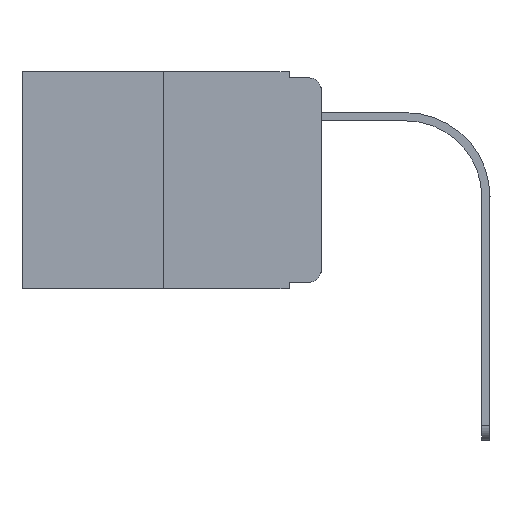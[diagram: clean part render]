
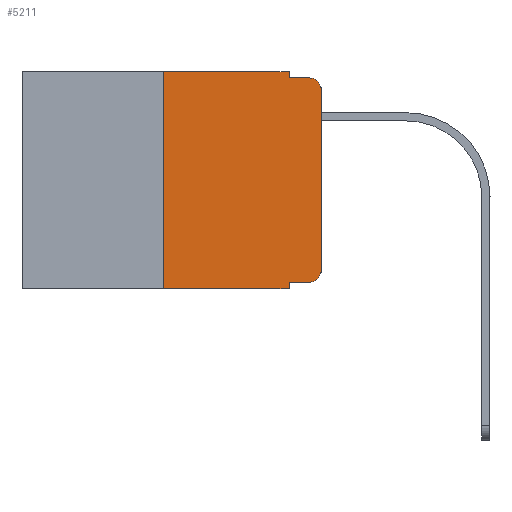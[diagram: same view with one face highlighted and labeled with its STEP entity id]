
A CAD part, left-side view. The second image highlights one B-rep face of the part: STEP entity #5211.
In plain terms, the highlighted planar face has unit normal (-1, 0, 0).
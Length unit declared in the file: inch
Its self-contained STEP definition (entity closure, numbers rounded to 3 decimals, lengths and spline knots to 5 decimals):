
#440 = CARTESIAN_POINT ( 'NONE',  ( 0., 0., -0.313 ) ) ;
#561 = AXIS2_PLACEMENT_3D ( 'NONE', #17655, #1024, #12655 ) ;
#601 = ORIENTED_EDGE ( 'NONE', *, *, #14092, .F. ) ;
#818 = VERTEX_POINT ( 'NONE', #8046 ) ;
#1024 = DIRECTION ( 'NONE',  ( -1., 0., 0. ) ) ;
#1051 = CARTESIAN_POINT ( 'NONE',  ( 0., 0., 0. ) ) ;
#1180 = CARTESIAN_POINT ( 'NONE',  ( 0., 0.473, -0.343 ) ) ;
#1638 = LINE ( 'NONE', #8075, #19813 ) ;
#1722 = DIRECTION ( 'NONE',  ( 0., -1., 0. ) ) ;
#1746 = PLANE ( 'NONE',  #20336 ) ;
#2055 = VECTOR ( 'NONE', #1722, 39.37008 ) ;
#2069 = CIRCLE ( 'NONE', #20827, 0.02 ) ;
#2169 = DIRECTION ( 'NONE',  ( -1., 0., 0. ) ) ;
#2252 = EDGE_CURVE ( 'NONE', #14280, #4525, #1638, .T. ) ;
#2274 = DIRECTION ( 'NONE',  ( 0., 0., -1. ) ) ;
#2506 = ORIENTED_EDGE ( 'NONE', *, *, #7189, .F. ) ;
#2559 = VERTEX_POINT ( 'NONE', #4293 ) ;
#2685 = CIRCLE ( 'NONE', #561, 0.02 ) ;
#2992 = CARTESIAN_POINT ( 'NONE',  ( 0., 0.02, -0.01 ) ) ;
#3070 = LINE ( 'NONE', #1180, #16499 ) ;
#3268 = ORIENTED_EDGE ( 'NONE', *, *, #11568, .T. ) ;
#3334 = VERTEX_POINT ( 'NONE', #2992 ) ;
#3627 = DIRECTION ( 'NONE',  ( 1., 0., 0. ) ) ;
#3714 = DIRECTION ( 'NONE',  ( 0., -1., 0. ) ) ;
#4293 = CARTESIAN_POINT ( 'NONE',  ( 0., 0.051, -0.333 ) ) ;
#4525 = VERTEX_POINT ( 'NONE', #16077 ) ;
#4785 = LINE ( 'NONE', #19764, #8509 ) ;
#5066 = FACE_OUTER_BOUND ( 'NONE', #5644, .T. ) ;
#5211 = ADVANCED_FACE ( 'NONE', ( #5066 ), #1746, .F. ) ;
#5538 = VECTOR ( 'NONE', #21335, 39.37008 ) ;
#5597 = VECTOR ( 'NONE', #10982, 39.37008 ) ;
#5644 = EDGE_LOOP ( 'NONE', ( #15351, #9209, #18653, #2506, #6189, #14084, #3268, #601, #20754, #16075 ) ) ;
#6189 = ORIENTED_EDGE ( 'NONE', *, *, #18873, .F. ) ;
#6763 = VERTEX_POINT ( 'NONE', #13357 ) ;
#7189 = EDGE_CURVE ( 'NONE', #19261, #6763, #21232, .T. ) ;
#7575 = VERTEX_POINT ( 'NONE', #15999 ) ;
#7802 = DIRECTION ( 'NONE',  ( 0., 0., 1. ) ) ;
#8043 = CARTESIAN_POINT ( 'NONE',  ( 0., 0.051, -0.333 ) ) ;
#8046 = CARTESIAN_POINT ( 'NONE',  ( 0., 0., -0.03 ) ) ;
#8075 = CARTESIAN_POINT ( 'NONE',  ( 0., 0.25, 0. ) ) ;
#8509 = VECTOR ( 'NONE', #21628, 39.37008 ) ;
#8555 = EDGE_CURVE ( 'NONE', #2559, #15479, #16454, .T. ) ;
#9209 = ORIENTED_EDGE ( 'NONE', *, *, #18903, .T. ) ;
#9537 = VERTEX_POINT ( 'NONE', #440 ) ;
#10046 = DIRECTION ( 'NONE',  ( 0., 0., -1. ) ) ;
#10611 = EDGE_CURVE ( 'NONE', #15479, #9537, #2685, .T. ) ;
#10982 = DIRECTION ( 'NONE',  ( 0., 0., -1. ) ) ;
#11568 = EDGE_CURVE ( 'NONE', #14280, #7575, #3070, .T. ) ;
#12121 = LINE ( 'NONE', #12356, #19756 ) ;
#12287 = VECTOR ( 'NONE', #7802, 39.37008 ) ;
#12356 = CARTESIAN_POINT ( 'NONE',  ( 0., 0.473, 0. ) ) ;
#12655 = DIRECTION ( 'NONE',  ( 0., 0., -1. ) ) ;
#13357 = CARTESIAN_POINT ( 'NONE',  ( 0., 0.051, -0.01 ) ) ;
#13408 = CARTESIAN_POINT ( 'NONE',  ( 0., 0.02, -0.333 ) ) ;
#13578 = CARTESIAN_POINT ( 'NONE',  ( 0., 0.473, 0. ) ) ;
#13600 = CARTESIAN_POINT ( 'NONE',  ( 0., 0.25, -0.343 ) ) ;
#14084 = ORIENTED_EDGE ( 'NONE', *, *, #2252, .F. ) ;
#14092 = EDGE_CURVE ( 'NONE', #2559, #7575, #17953, .T. ) ;
#14280 = VERTEX_POINT ( 'NONE', #13600 ) ;
#14578 = CARTESIAN_POINT ( 'NONE',  ( 0., 0.051, 0. ) ) ;
#14737 = CARTESIAN_POINT ( 'NONE',  ( 0., 0.051, 0. ) ) ;
#15351 = ORIENTED_EDGE ( 'NONE', *, *, #17913, .T. ) ;
#15479 = VERTEX_POINT ( 'NONE', #13408 ) ;
#15999 = CARTESIAN_POINT ( 'NONE',  ( 0., 0.051, -0.343 ) ) ;
#16075 = ORIENTED_EDGE ( 'NONE', *, *, #10611, .T. ) ;
#16077 = CARTESIAN_POINT ( 'NONE',  ( 0., 0.25, 0. ) ) ;
#16454 = LINE ( 'NONE', #8043, #2055 ) ;
#16499 = VECTOR ( 'NONE', #21463, 39.37008 ) ;
#16608 = DIRECTION ( 'NONE',  ( 0., 0., 1. ) ) ;
#17655 = CARTESIAN_POINT ( 'NONE',  ( 0., 0.02, -0.313 ) ) ;
#17913 = EDGE_CURVE ( 'NONE', #9537, #818, #17998, .T. ) ;
#17953 = LINE ( 'NONE', #14737, #5597 ) ;
#17998 = LINE ( 'NONE', #1051, #12287 ) ;
#18653 = ORIENTED_EDGE ( 'NONE', *, *, #21869, .F. ) ;
#18873 = EDGE_CURVE ( 'NONE', #4525, #19261, #12121, .T. ) ;
#18903 = EDGE_CURVE ( 'NONE', #818, #3334, #2069, .T. ) ;
#19228 = CARTESIAN_POINT ( 'NONE',  ( 0., 0.02, -0.03 ) ) ;
#19261 = VERTEX_POINT ( 'NONE', #19956 ) ;
#19756 = VECTOR ( 'NONE', #3714, 39.37008 ) ;
#19764 = CARTESIAN_POINT ( 'NONE',  ( 0., 0.051, -0.01 ) ) ;
#19813 = VECTOR ( 'NONE', #16608, 39.37008 ) ;
#19956 = CARTESIAN_POINT ( 'NONE',  ( 0., 0.051, 0. ) ) ;
#20336 = AXIS2_PLACEMENT_3D ( 'NONE', #13578, #3627, #10046 ) ;
#20754 = ORIENTED_EDGE ( 'NONE', *, *, #8555, .T. ) ;
#20827 = AXIS2_PLACEMENT_3D ( 'NONE', #19228, #2169, #2274 ) ;
#21232 = LINE ( 'NONE', #14578, #5538 ) ;
#21335 = DIRECTION ( 'NONE',  ( 0., 0., -1. ) ) ;
#21463 = DIRECTION ( 'NONE',  ( 0., -1., 0. ) ) ;
#21628 = DIRECTION ( 'NONE',  ( 0., -1., 0. ) ) ;
#21869 = EDGE_CURVE ( 'NONE', #6763, #3334, #4785, .T. ) ;
